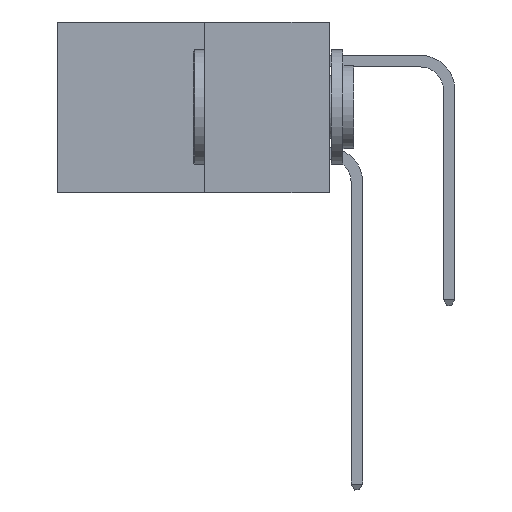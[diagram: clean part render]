
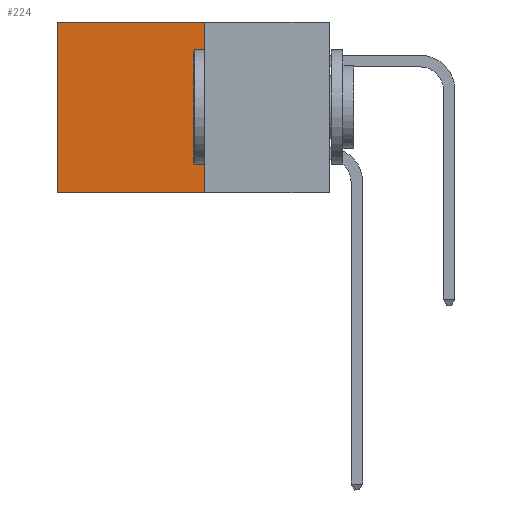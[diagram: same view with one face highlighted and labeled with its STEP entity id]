
A CAD part, left-side view. The second image highlights one B-rep face of the part: STEP entity #224.
In plain terms, the highlighted planar face has unit normal (-1, 0, 0).
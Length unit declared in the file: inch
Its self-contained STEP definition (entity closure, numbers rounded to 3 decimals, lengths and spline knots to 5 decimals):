
#109 = CARTESIAN_POINT ( 'NONE',  ( 0.277, 0.27, -0.37 ) ) ;
#224 = ADVANCED_FACE ( 'NONE', ( #674 ), #25010, .F. ) ;
#674 = FACE_OUTER_BOUND ( 'NONE', #16354, .T. ) ;
#932 = DIRECTION ( 'NONE',  ( 1., 0., 0. ) ) ;
#1167 = VECTOR ( 'NONE', #16862, 39.37008 ) ;
#1552 = ORIENTED_EDGE ( 'NONE', *, *, #9055, .T. ) ;
#2533 = VERTEX_POINT ( 'NONE', #109 ) ;
#5937 = EDGE_CURVE ( 'NONE', #10928, #22799, #15034, .T. ) ;
#6242 = LINE ( 'NONE', #24150, #17785 ) ;
#7209 = LINE ( 'NONE', #24899, #12625 ) ;
#7596 = ORIENTED_EDGE ( 'NONE', *, *, #12182, .F. ) ;
#8276 = EDGE_CURVE ( 'NONE', #2533, #22799, #21038, .T. ) ;
#8336 = CARTESIAN_POINT ( 'NONE',  ( 0.277, 0.27, -0.37 ) ) ;
#8394 = DIRECTION ( 'NONE',  ( 0., 1., 0. ) ) ;
#9055 = EDGE_CURVE ( 'NONE', #21575, #10928, #6242, .T. ) ;
#9395 = CARTESIAN_POINT ( 'NONE',  ( 0.277, 0.59, 0. ) ) ;
#10276 = VECTOR ( 'NONE', #8394, 39.37008 ) ;
#10928 = VERTEX_POINT ( 'NONE', #9395 ) ;
#12182 = EDGE_CURVE ( 'NONE', #21575, #2533, #7209, .T. ) ;
#12625 = VECTOR ( 'NONE', #13478, 39.37008 ) ;
#13307 = CARTESIAN_POINT ( 'NONE',  ( 0.277, 0.59, -0.37 ) ) ;
#13478 = DIRECTION ( 'NONE',  ( 0., 0., -1. ) ) ;
#14284 = ORIENTED_EDGE ( 'NONE', *, *, #5937, .T. ) ;
#14890 = CARTESIAN_POINT ( 'NONE',  ( 0.277, 0.27, -0.37 ) ) ;
#15034 = LINE ( 'NONE', #17396, #1167 ) ;
#16354 = EDGE_LOOP ( 'NONE', ( #14284, #24142, #7596, #1552 ) ) ;
#16862 = DIRECTION ( 'NONE',  ( 0., 0., -1. ) ) ;
#17396 = CARTESIAN_POINT ( 'NONE',  ( 0.277, 0.59, -0.37 ) ) ;
#17785 = VECTOR ( 'NONE', #23097, 39.37008 ) ;
#21038 = LINE ( 'NONE', #8336, #10276 ) ;
#21104 = AXIS2_PLACEMENT_3D ( 'NONE', #14890, #932, #27277 ) ;
#21575 = VERTEX_POINT ( 'NONE', #22691 ) ;
#22691 = CARTESIAN_POINT ( 'NONE',  ( 0.277, 0.27, 0. ) ) ;
#22799 = VERTEX_POINT ( 'NONE', #13307 ) ;
#23097 = DIRECTION ( 'NONE',  ( 0., 1., 0. ) ) ;
#24142 = ORIENTED_EDGE ( 'NONE', *, *, #8276, .F. ) ;
#24150 = CARTESIAN_POINT ( 'NONE',  ( 0.277, 0.27, 0. ) ) ;
#24899 = CARTESIAN_POINT ( 'NONE',  ( 0.277, 0.27, -0.37 ) ) ;
#25010 = PLANE ( 'NONE',  #21104 ) ;
#27277 = DIRECTION ( 'NONE',  ( 0., 0., -1. ) ) ;
